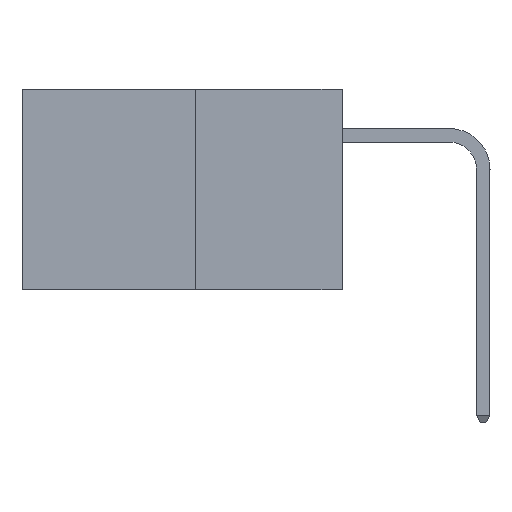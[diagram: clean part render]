
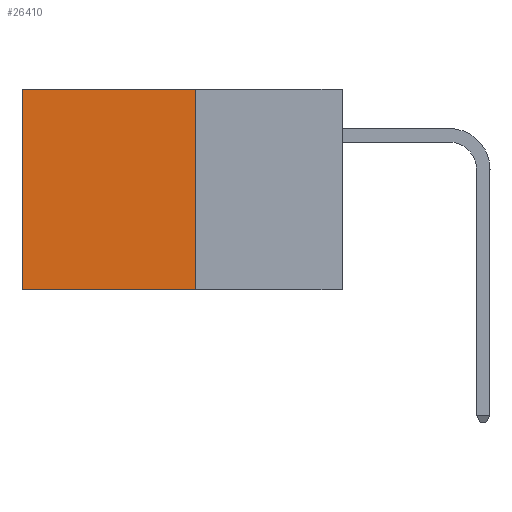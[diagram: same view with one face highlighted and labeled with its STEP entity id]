
A CAD part, left-side view. The second image highlights one B-rep face of the part: STEP entity #26410.
In plain terms, the highlighted planar face has unit normal (-1, 0, 0).
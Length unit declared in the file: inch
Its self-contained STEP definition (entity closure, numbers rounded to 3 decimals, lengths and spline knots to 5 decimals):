
#1564 = LINE ( 'NONE', #1904, #7072 ) ;
#1904 = CARTESIAN_POINT ( 'NONE',  ( 0.277, 0.27, -0.37 ) ) ;
#2010 = DIRECTION ( 'NONE',  ( 0., 0., -1. ) ) ;
#2808 = EDGE_LOOP ( 'NONE', ( #20305, #18307, #8384, #11114 ) ) ;
#5367 = DIRECTION ( 'NONE',  ( 0., 0., -1. ) ) ;
#5548 = EDGE_CURVE ( 'NONE', #10458, #19765, #21889, .T. ) ;
#6758 = CARTESIAN_POINT ( 'NONE',  ( 0.277, 0.27, -0.37 ) ) ;
#7072 = VECTOR ( 'NONE', #14169, 39.37008 ) ;
#7428 = EDGE_CURVE ( 'NONE', #19765, #12412, #1564, .T. ) ;
#8384 = ORIENTED_EDGE ( 'NONE', *, *, #5548, .F. ) ;
#9155 = EDGE_CURVE ( 'NONE', #11600, #12412, #12398, .T. ) ;
#9221 = FACE_OUTER_BOUND ( 'NONE', #2808, .T. ) ;
#10373 = VECTOR ( 'NONE', #20514, 39.37008 ) ;
#10458 = VERTEX_POINT ( 'NONE', #19446 ) ;
#10874 = CARTESIAN_POINT ( 'NONE',  ( 0.277, 0.59, -0.37 ) ) ;
#11114 = ORIENTED_EDGE ( 'NONE', *, *, #16532, .T. ) ;
#11520 = AXIS2_PLACEMENT_3D ( 'NONE', #12239, #14270, #2010 ) ;
#11600 = VERTEX_POINT ( 'NONE', #25061 ) ;
#12239 = CARTESIAN_POINT ( 'NONE',  ( 0.277, 0.27, -0.37 ) ) ;
#12398 = LINE ( 'NONE', #15461, #22629 ) ;
#12412 = VERTEX_POINT ( 'NONE', #10874 ) ;
#12844 = DIRECTION ( 'NONE',  ( 0., 1., 0. ) ) ;
#14169 = DIRECTION ( 'NONE',  ( 0., 1., 0. ) ) ;
#14270 = DIRECTION ( 'NONE',  ( 1., 0., 0. ) ) ;
#15461 = CARTESIAN_POINT ( 'NONE',  ( 0.277, 0.59, -0.37 ) ) ;
#16532 = EDGE_CURVE ( 'NONE', #10458, #11600, #18385, .T. ) ;
#17744 = VECTOR ( 'NONE', #12844, 39.37008 ) ;
#18307 = ORIENTED_EDGE ( 'NONE', *, *, #7428, .F. ) ;
#18385 = LINE ( 'NONE', #20989, #17744 ) ;
#19446 = CARTESIAN_POINT ( 'NONE',  ( 0.277, 0.27, 0. ) ) ;
#19765 = VERTEX_POINT ( 'NONE', #19990 ) ;
#19990 = CARTESIAN_POINT ( 'NONE',  ( 0.277, 0.27, -0.37 ) ) ;
#20305 = ORIENTED_EDGE ( 'NONE', *, *, #9155, .T. ) ;
#20514 = DIRECTION ( 'NONE',  ( 0., 0., -1. ) ) ;
#20989 = CARTESIAN_POINT ( 'NONE',  ( 0.277, 0.27, 0. ) ) ;
#21889 = LINE ( 'NONE', #6758, #10373 ) ;
#22629 = VECTOR ( 'NONE', #5367, 39.37008 ) ;
#24502 = PLANE ( 'NONE',  #11520 ) ;
#25061 = CARTESIAN_POINT ( 'NONE',  ( 0.277, 0.59, 0. ) ) ;
#26410 = ADVANCED_FACE ( 'NONE', ( #9221 ), #24502, .F. ) ;
